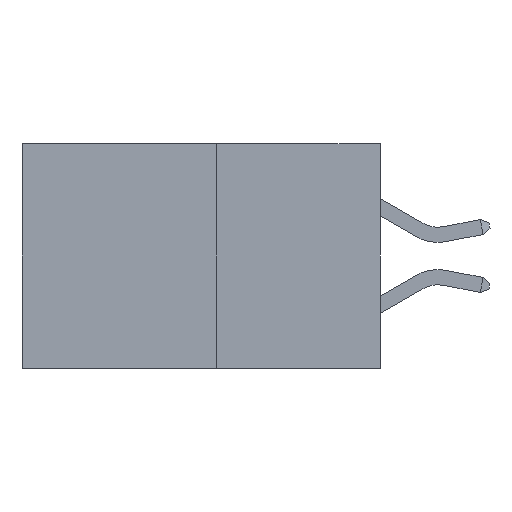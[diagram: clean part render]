
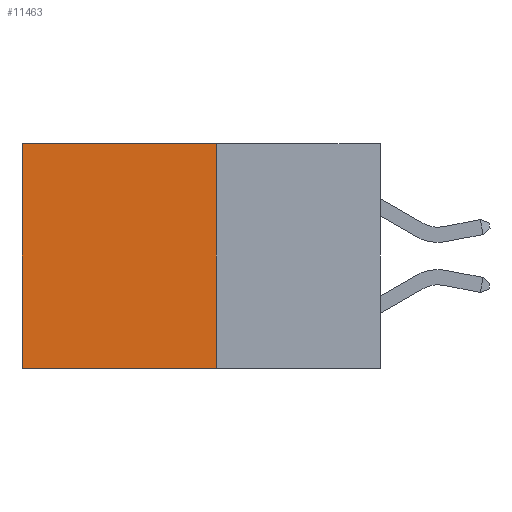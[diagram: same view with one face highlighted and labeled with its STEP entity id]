
A CAD part, left-side view. The second image highlights one B-rep face of the part: STEP entity #11463.
In plain terms, the highlighted planar face has unit normal (-1, 0, 0).
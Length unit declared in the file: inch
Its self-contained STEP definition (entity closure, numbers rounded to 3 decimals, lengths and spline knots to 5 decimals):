
#45 = VECTOR ( 'NONE', #9799, 39.37008 ) ;
#246 = EDGE_CURVE ( 'NONE', #4767, #9625, #12477, .T. ) ;
#968 = FACE_OUTER_BOUND ( 'NONE', #2173, .T. ) ;
#1128 = CARTESIAN_POINT ( 'NONE',  ( 0.277, 0.59, -0.37 ) ) ;
#1135 = CARTESIAN_POINT ( 'NONE',  ( 0.277, 0.59, 0. ) ) ;
#1280 = EDGE_CURVE ( 'NONE', #4767, #5831, #6503, .T. ) ;
#1309 = CARTESIAN_POINT ( 'NONE',  ( 0.277, 0.27, 0. ) ) ;
#2173 = EDGE_LOOP ( 'NONE', ( #4308, #7898, #5879, #9433 ) ) ;
#2251 = LINE ( 'NONE', #11436, #7517 ) ;
#2579 = DIRECTION ( 'NONE',  ( 0., 1., 0. ) ) ;
#2860 = CARTESIAN_POINT ( 'NONE',  ( 0.277, 0.59, -0.37 ) ) ;
#3295 = PLANE ( 'NONE',  #4548 ) ;
#4282 = CARTESIAN_POINT ( 'NONE',  ( 0.277, 0.27, -0.37 ) ) ;
#4308 = ORIENTED_EDGE ( 'NONE', *, *, #8256, .T. ) ;
#4548 = AXIS2_PLACEMENT_3D ( 'NONE', #4282, #5295, #12172 ) ;
#4767 = VERTEX_POINT ( 'NONE', #9962 ) ;
#4952 = LINE ( 'NONE', #2860, #45 ) ;
#5080 = DIRECTION ( 'NONE',  ( 0., 0., -1. ) ) ;
#5295 = DIRECTION ( 'NONE',  ( 1., 0., 0. ) ) ;
#5440 = DIRECTION ( 'NONE',  ( 0., 1., 0. ) ) ;
#5776 = EDGE_CURVE ( 'NONE', #5831, #10649, #2251, .T. ) ;
#5831 = VERTEX_POINT ( 'NONE', #10509 ) ;
#5879 = ORIENTED_EDGE ( 'NONE', *, *, #1280, .F. ) ;
#6312 = CARTESIAN_POINT ( 'NONE',  ( 0.277, 0.27, -0.37 ) ) ;
#6503 = LINE ( 'NONE', #6312, #9733 ) ;
#7517 = VECTOR ( 'NONE', #2579, 39.37008 ) ;
#7898 = ORIENTED_EDGE ( 'NONE', *, *, #5776, .F. ) ;
#8256 = EDGE_CURVE ( 'NONE', #9625, #10649, #4952, .T. ) ;
#9433 = ORIENTED_EDGE ( 'NONE', *, *, #246, .T. ) ;
#9625 = VERTEX_POINT ( 'NONE', #1135 ) ;
#9733 = VECTOR ( 'NONE', #5080, 39.37008 ) ;
#9799 = DIRECTION ( 'NONE',  ( 0., 0., -1. ) ) ;
#9962 = CARTESIAN_POINT ( 'NONE',  ( 0.277, 0.27, 0. ) ) ;
#10509 = CARTESIAN_POINT ( 'NONE',  ( 0.277, 0.27, -0.37 ) ) ;
#10649 = VERTEX_POINT ( 'NONE', #1128 ) ;
#11436 = CARTESIAN_POINT ( 'NONE',  ( 0.277, 0.27, -0.37 ) ) ;
#11463 = ADVANCED_FACE ( 'NONE', ( #968 ), #3295, .F. ) ;
#12172 = DIRECTION ( 'NONE',  ( 0., 0., -1. ) ) ;
#12180 = VECTOR ( 'NONE', #5440, 39.37008 ) ;
#12477 = LINE ( 'NONE', #1309, #12180 ) ;
